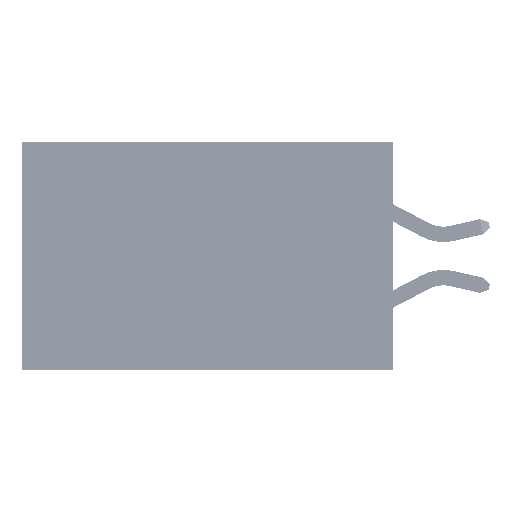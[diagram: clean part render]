
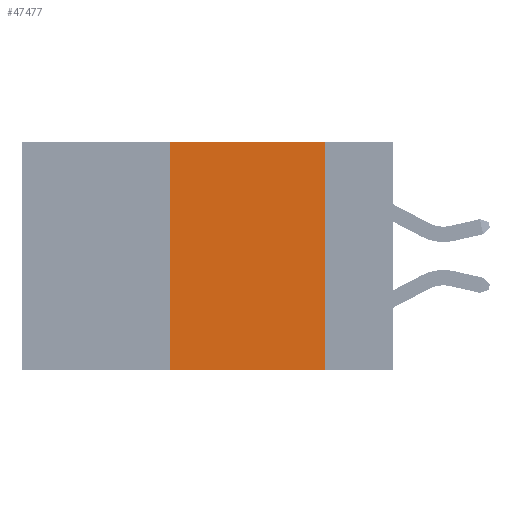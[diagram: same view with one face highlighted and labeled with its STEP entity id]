
A CAD part, left-side view. The second image highlights one B-rep face of the part: STEP entity #47477.
In plain terms, the highlighted planar face has unit normal (-1, 0, 0).
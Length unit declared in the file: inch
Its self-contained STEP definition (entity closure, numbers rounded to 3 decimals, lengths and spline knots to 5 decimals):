
#1762 = CARTESIAN_POINT ( 'NONE',  ( 0., 0.6, 0. ) ) ;
#2867 = ORIENTED_EDGE ( 'NONE', *, *, #5049, .F. ) ;
#5049 = EDGE_CURVE ( 'NONE', #40474, #15467, #31188, .T. ) ;
#5147 = AXIS2_PLACEMENT_3D ( 'NONE', #38456, #31303, #16512 ) ;
#6405 = CARTESIAN_POINT ( 'NONE',  ( 0., 0.11, 0. ) ) ;
#6465 = EDGE_CURVE ( 'NONE', #37879, #6981, #31673, .T. ) ;
#6981 = VERTEX_POINT ( 'NONE', #32354 ) ;
#8729 = CARTESIAN_POINT ( 'NONE',  ( 0., 0.11, 0. ) ) ;
#9507 = EDGE_CURVE ( 'NONE', #37879, #15467, #12019, .T. ) ;
#12019 = LINE ( 'NONE', #34227, #39096 ) ;
#12645 = DIRECTION ( 'NONE',  ( 0., -1., 0. ) ) ;
#12960 = VECTOR ( 'NONE', #19607, 39.37008 ) ;
#15467 = VERTEX_POINT ( 'NONE', #44560 ) ;
#16512 = DIRECTION ( 'NONE',  ( 0., 0., -1. ) ) ;
#16844 = LINE ( 'NONE', #1762, #22942 ) ;
#19607 = DIRECTION ( 'NONE',  ( 0., 0., -1. ) ) ;
#22624 = CARTESIAN_POINT ( 'NONE',  ( 0., 0.36, -0.37 ) ) ;
#22942 = VECTOR ( 'NONE', #12645, 39.37008 ) ;
#23324 = DIRECTION ( 'NONE',  ( 0., 0., 1. ) ) ;
#27136 = FACE_OUTER_BOUND ( 'NONE', #31762, .T. ) ;
#30587 = ORIENTED_EDGE ( 'NONE', *, *, #9507, .T. ) ;
#30672 = ORIENTED_EDGE ( 'NONE', *, *, #34010, .F. ) ;
#31188 = LINE ( 'NONE', #8729, #12960 ) ;
#31303 = DIRECTION ( 'NONE',  ( 1., 0., 0. ) ) ;
#31673 = LINE ( 'NONE', #46456, #41411 ) ;
#31762 = EDGE_LOOP ( 'NONE', ( #2867, #30672, #38473, #30587 ) ) ;
#32354 = CARTESIAN_POINT ( 'NONE',  ( 0., 0.36, 0. ) ) ;
#34010 = EDGE_CURVE ( 'NONE', #6981, #40474, #16844, .T. ) ;
#34227 = CARTESIAN_POINT ( 'NONE',  ( 0., 0.6, -0.37 ) ) ;
#37879 = VERTEX_POINT ( 'NONE', #22624 ) ;
#38396 = DIRECTION ( 'NONE',  ( 0., -1., 0. ) ) ;
#38456 = CARTESIAN_POINT ( 'NONE',  ( 0., 0.6, 0. ) ) ;
#38473 = ORIENTED_EDGE ( 'NONE', *, *, #6465, .F. ) ;
#39096 = VECTOR ( 'NONE', #38396, 39.37008 ) ;
#40474 = VERTEX_POINT ( 'NONE', #6405 ) ;
#41411 = VECTOR ( 'NONE', #23324, 39.37008 ) ;
#44560 = CARTESIAN_POINT ( 'NONE',  ( 0., 0.11, -0.37 ) ) ;
#46456 = CARTESIAN_POINT ( 'NONE',  ( 0., 0.36, 0. ) ) ;
#46570 = PLANE ( 'NONE',  #5147 ) ;
#47477 = ADVANCED_FACE ( 'NONE', ( #27136 ), #46570, .F. ) ;
